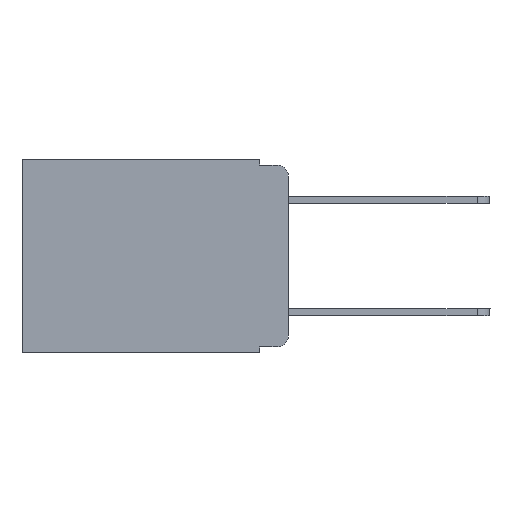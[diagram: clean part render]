
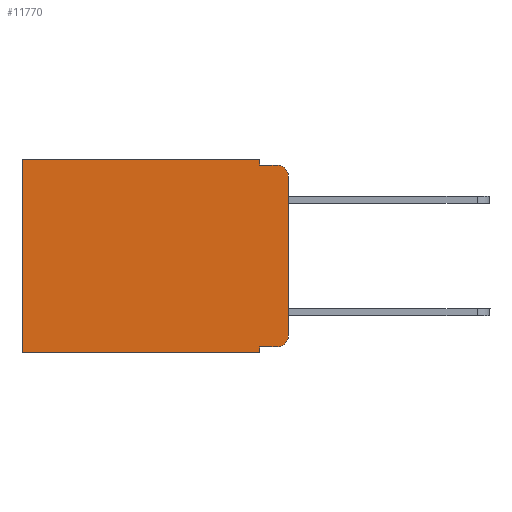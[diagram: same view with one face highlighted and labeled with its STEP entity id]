
A CAD part, left-side view. The second image highlights one B-rep face of the part: STEP entity #11770.
In plain terms, the highlighted planar face has unit normal (-1, 0, 0).
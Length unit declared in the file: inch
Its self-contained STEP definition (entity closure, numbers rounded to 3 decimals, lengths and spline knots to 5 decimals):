
#279 = LINE ( 'NONE', #2562, #6808 ) ;
#510 = VERTEX_POINT ( 'NONE', #4868 ) ;
#625 = EDGE_CURVE ( 'NONE', #510, #9271, #12042, .T. ) ;
#1043 = AXIS2_PLACEMENT_3D ( 'NONE', #2386, #1456, #5406 ) ;
#1147 = CARTESIAN_POINT ( 'NONE',  ( 0.298, 0.473, -0.343 ) ) ;
#1205 = FACE_OUTER_BOUND ( 'NONE', #6046, .T. ) ;
#1456 = DIRECTION ( 'NONE',  ( -1., 0., 0. ) ) ;
#1684 = VERTEX_POINT ( 'NONE', #12526 ) ;
#1911 = EDGE_CURVE ( 'NONE', #9178, #2527, #12347, .T. ) ;
#2127 = CARTESIAN_POINT ( 'NONE',  ( 0.298, 0.051, -0.333 ) ) ;
#2384 = LINE ( 'NONE', #3521, #9382 ) ;
#2386 = CARTESIAN_POINT ( 'NONE',  ( 0.298, 0.02, -0.03 ) ) ;
#2527 = VERTEX_POINT ( 'NONE', #9223 ) ;
#2558 = PLANE ( 'NONE',  #4177 ) ;
#2562 = CARTESIAN_POINT ( 'NONE',  ( 0.298, 0., 0. ) ) ;
#2638 = ORIENTED_EDGE ( 'NONE', *, *, #13179, .T. ) ;
#2949 = CARTESIAN_POINT ( 'NONE',  ( 0.298, 0., 0. ) ) ;
#3440 = DIRECTION ( 'NONE',  ( 0., 0., -1. ) ) ;
#3521 = CARTESIAN_POINT ( 'NONE',  ( 0.298, 0., -0.343 ) ) ;
#3760 = DIRECTION ( 'NONE',  ( 0., 0., -1. ) ) ;
#4177 = AXIS2_PLACEMENT_3D ( 'NONE', #10812, #10692, #5718 ) ;
#4414 = CARTESIAN_POINT ( 'NONE',  ( 0.298, 0.473, 0. ) ) ;
#4445 = DIRECTION ( 'NONE',  ( 0., -1., 0. ) ) ;
#4623 = LINE ( 'NONE', #12842, #5393 ) ;
#4804 = VERTEX_POINT ( 'NONE', #7440 ) ;
#4868 = CARTESIAN_POINT ( 'NONE',  ( 0.298, 0.473, 0. ) ) ;
#5126 = ORIENTED_EDGE ( 'NONE', *, *, #10670, .T. ) ;
#5307 = EDGE_CURVE ( 'NONE', #1684, #7682, #4623, .T. ) ;
#5393 = VECTOR ( 'NONE', #5460, 39.37008 ) ;
#5406 = DIRECTION ( 'NONE',  ( 0., 0., -1. ) ) ;
#5460 = DIRECTION ( 'NONE',  ( 0., 0., -1. ) ) ;
#5465 = VERTEX_POINT ( 'NONE', #12344 ) ;
#5607 = CIRCLE ( 'NONE', #11307, 0.02 ) ;
#5667 = VERTEX_POINT ( 'NONE', #12574 ) ;
#5718 = DIRECTION ( 'NONE',  ( 0., 0., -1. ) ) ;
#6046 = EDGE_LOOP ( 'NONE', ( #9577, #6689, #9362, #7351, #5126, #11931, #9435, #9891, #2638, #10118 ) ) ;
#6080 = DIRECTION ( 'NONE',  ( 0., 0., -1. ) ) ;
#6162 = VECTOR ( 'NONE', #10088, 39.37008 ) ;
#6513 = LINE ( 'NONE', #2949, #6162 ) ;
#6662 = VERTEX_POINT ( 'NONE', #12958 ) ;
#6689 = ORIENTED_EDGE ( 'NONE', *, *, #11679, .T. ) ;
#6714 = DIRECTION ( 'NONE',  ( 0., 1., 0. ) ) ;
#6808 = VECTOR ( 'NONE', #8599, 39.37008 ) ;
#7246 = CIRCLE ( 'NONE', #1043, 0.02 ) ;
#7351 = ORIENTED_EDGE ( 'NONE', *, *, #5307, .F. ) ;
#7440 = CARTESIAN_POINT ( 'NONE',  ( 0.298, 0.02, -0.333 ) ) ;
#7682 = VERTEX_POINT ( 'NONE', #7939 ) ;
#7869 = DIRECTION ( 'NONE',  ( -1., 0., 0. ) ) ;
#7939 = CARTESIAN_POINT ( 'NONE',  ( 0.298, 0.051, -0.01 ) ) ;
#8582 = LINE ( 'NONE', #11130, #10190 ) ;
#8599 = DIRECTION ( 'NONE',  ( 0., 1., 0. ) ) ;
#8810 = VECTOR ( 'NONE', #10005, 39.37008 ) ;
#9038 = CARTESIAN_POINT ( 'NONE',  ( 0.298, 0.051, -0.333 ) ) ;
#9178 = VERTEX_POINT ( 'NONE', #2127 ) ;
#9223 = CARTESIAN_POINT ( 'NONE',  ( 0.298, 0.051, -0.343 ) ) ;
#9271 = VERTEX_POINT ( 'NONE', #1147 ) ;
#9362 = ORIENTED_EDGE ( 'NONE', *, *, #9790, .F. ) ;
#9382 = VECTOR ( 'NONE', #6714, 39.37008 ) ;
#9435 = ORIENTED_EDGE ( 'NONE', *, *, #9797, .F. ) ;
#9577 = ORIENTED_EDGE ( 'NONE', *, *, #9770, .F. ) ;
#9770 = EDGE_CURVE ( 'NONE', #6662, #5465, #6513, .T. ) ;
#9790 = EDGE_CURVE ( 'NONE', #7682, #5667, #8582, .T. ) ;
#9797 = EDGE_CURVE ( 'NONE', #2527, #9271, #2384, .T. ) ;
#9891 = ORIENTED_EDGE ( 'NONE', *, *, #1911, .F. ) ;
#9921 = VECTOR ( 'NONE', #3440, 39.37008 ) ;
#9930 = CARTESIAN_POINT ( 'NONE',  ( 0.298, 0.02, -0.313 ) ) ;
#10005 = DIRECTION ( 'NONE',  ( 0., -1., 0. ) ) ;
#10088 = DIRECTION ( 'NONE',  ( 0., 0., -1. ) ) ;
#10118 = ORIENTED_EDGE ( 'NONE', *, *, #12510, .T. ) ;
#10190 = VECTOR ( 'NONE', #4445, 39.37008 ) ;
#10670 = EDGE_CURVE ( 'NONE', #1684, #510, #279, .T. ) ;
#10692 = DIRECTION ( 'NONE',  ( 1., 0., 0. ) ) ;
#10812 = CARTESIAN_POINT ( 'NONE',  ( 0.298, 0., 0. ) ) ;
#11130 = CARTESIAN_POINT ( 'NONE',  ( 0.298, 0.051, -0.01 ) ) ;
#11307 = AXIS2_PLACEMENT_3D ( 'NONE', #9930, #7869, #3760 ) ;
#11582 = LINE ( 'NONE', #9038, #8810 ) ;
#11679 = EDGE_CURVE ( 'NONE', #6662, #5667, #7246, .T. ) ;
#11770 = ADVANCED_FACE ( 'NONE', ( #1205 ), #2558, .F. ) ;
#11931 = ORIENTED_EDGE ( 'NONE', *, *, #625, .T. ) ;
#12042 = LINE ( 'NONE', #4414, #9921 ) ;
#12283 = CARTESIAN_POINT ( 'NONE',  ( 0.298, 0.051, 0. ) ) ;
#12344 = CARTESIAN_POINT ( 'NONE',  ( 0.298, 0., -0.313 ) ) ;
#12347 = LINE ( 'NONE', #12283, #12682 ) ;
#12510 = EDGE_CURVE ( 'NONE', #4804, #5465, #5607, .T. ) ;
#12526 = CARTESIAN_POINT ( 'NONE',  ( 0.298, 0.051, 0. ) ) ;
#12574 = CARTESIAN_POINT ( 'NONE',  ( 0.298, 0.02, -0.01 ) ) ;
#12682 = VECTOR ( 'NONE', #6080, 39.37008 ) ;
#12842 = CARTESIAN_POINT ( 'NONE',  ( 0.298, 0.051, 0. ) ) ;
#12958 = CARTESIAN_POINT ( 'NONE',  ( 0.298, 0., -0.03 ) ) ;
#13179 = EDGE_CURVE ( 'NONE', #9178, #4804, #11582, .T. ) ;
